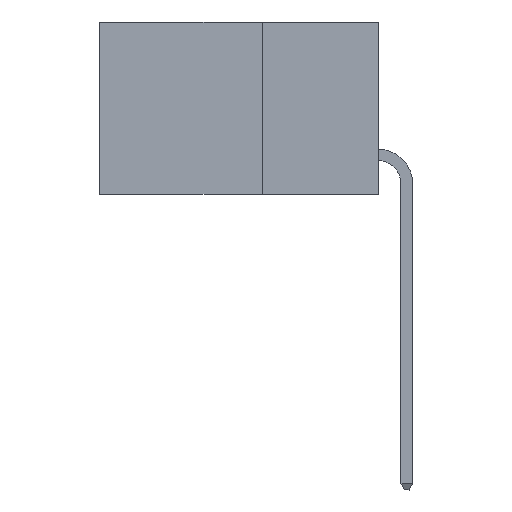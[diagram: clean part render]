
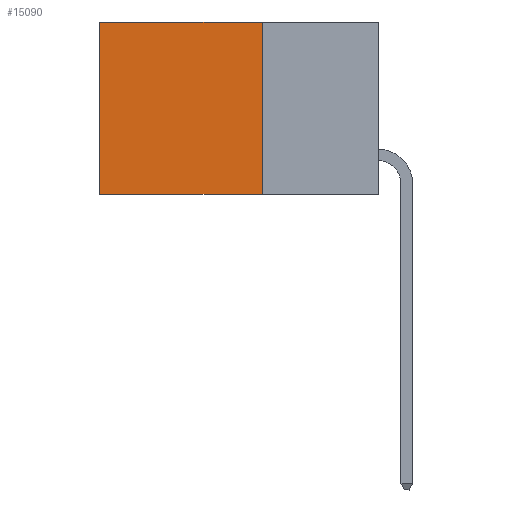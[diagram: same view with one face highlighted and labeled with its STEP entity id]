
A CAD part, left-side view. The second image highlights one B-rep face of the part: STEP entity #15090.
In plain terms, the highlighted planar face has unit normal (-1, 0, 0).
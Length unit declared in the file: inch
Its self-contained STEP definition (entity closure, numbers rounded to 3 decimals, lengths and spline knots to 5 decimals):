
#62 = CARTESIAN_POINT ( 'NONE',  ( 0.298, 0.25, 0. ) ) ;
#384 = ORIENTED_EDGE ( 'NONE', *, *, #14470, .F. ) ;
#385 = FACE_OUTER_BOUND ( 'NONE', #12048, .T. ) ;
#858 = CARTESIAN_POINT ( 'NONE',  ( 0.298, 0.6, 0. ) ) ;
#875 = VECTOR ( 'NONE', #7869, 39.37008 ) ;
#1184 = EDGE_CURVE ( 'NONE', #8060, #8944, #14808, .T. ) ;
#1221 = LINE ( 'NONE', #4078, #7064 ) ;
#1487 = CARTESIAN_POINT ( 'NONE',  ( 0.298, 0.25, 0. ) ) ;
#1617 = PLANE ( 'NONE',  #12684 ) ;
#1971 = VERTEX_POINT ( 'NONE', #4353 ) ;
#2366 = ORIENTED_EDGE ( 'NONE', *, *, #7037, .T. ) ;
#3811 = CARTESIAN_POINT ( 'NONE',  ( 0.298, 0.25, 0. ) ) ;
#4078 = CARTESIAN_POINT ( 'NONE',  ( 0.298, 0.25, -0.37 ) ) ;
#4353 = CARTESIAN_POINT ( 'NONE',  ( 0.298, 0.6, -0.37 ) ) ;
#5120 = DIRECTION ( 'NONE',  ( 1., 0., 0. ) ) ;
#6330 = LINE ( 'NONE', #858, #875 ) ;
#6874 = VERTEX_POINT ( 'NONE', #7553 ) ;
#7037 = EDGE_CURVE ( 'NONE', #8944, #1971, #6330, .T. ) ;
#7064 = VECTOR ( 'NONE', #13556, 39.37008 ) ;
#7553 = CARTESIAN_POINT ( 'NONE',  ( 0.298, 0.25, -0.37 ) ) ;
#7653 = CARTESIAN_POINT ( 'NONE',  ( 0.298, 0.6, 0. ) ) ;
#7736 = DIRECTION ( 'NONE',  ( 0., 1., 0. ) ) ;
#7869 = DIRECTION ( 'NONE',  ( 0., 0., -1. ) ) ;
#8060 = VERTEX_POINT ( 'NONE', #3811 ) ;
#8424 = ORIENTED_EDGE ( 'NONE', *, *, #1184, .T. ) ;
#8499 = DIRECTION ( 'NONE',  ( 0., 0., -1. ) ) ;
#8944 = VERTEX_POINT ( 'NONE', #7653 ) ;
#9241 = VECTOR ( 'NONE', #8499, 39.37008 ) ;
#11265 = VECTOR ( 'NONE', #7736, 39.37008 ) ;
#11793 = ORIENTED_EDGE ( 'NONE', *, *, #12264, .F. ) ;
#12048 = EDGE_LOOP ( 'NONE', ( #2366, #11793, #384, #8424 ) ) ;
#12231 = CARTESIAN_POINT ( 'NONE',  ( 0.298, 0.25, 0. ) ) ;
#12264 = EDGE_CURVE ( 'NONE', #6874, #1971, #1221, .T. ) ;
#12394 = LINE ( 'NONE', #1487, #9241 ) ;
#12684 = AXIS2_PLACEMENT_3D ( 'NONE', #12231, #5120, #13445 ) ;
#13445 = DIRECTION ( 'NONE',  ( 0., 0., -1. ) ) ;
#13556 = DIRECTION ( 'NONE',  ( 0., 1., 0. ) ) ;
#14470 = EDGE_CURVE ( 'NONE', #8060, #6874, #12394, .T. ) ;
#14808 = LINE ( 'NONE', #62, #11265 ) ;
#15090 = ADVANCED_FACE ( 'NONE', ( #385 ), #1617, .F. ) ;
